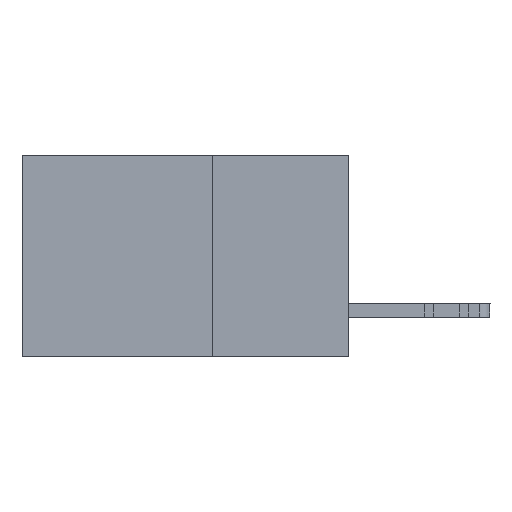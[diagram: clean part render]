
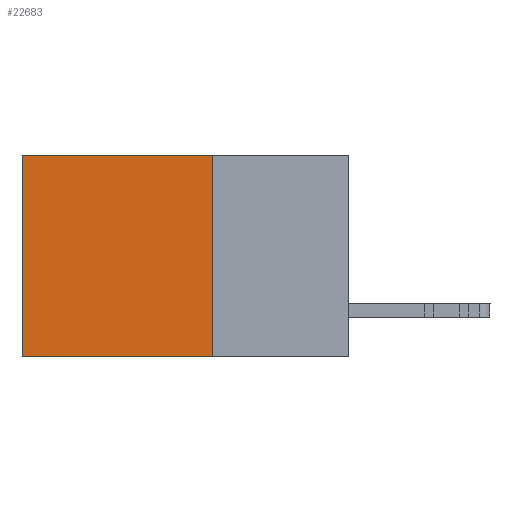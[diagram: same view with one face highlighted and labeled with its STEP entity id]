
A CAD part, left-side view. The second image highlights one B-rep face of the part: STEP entity #22683.
In plain terms, the highlighted planar face has unit normal (-1, 0, 0).
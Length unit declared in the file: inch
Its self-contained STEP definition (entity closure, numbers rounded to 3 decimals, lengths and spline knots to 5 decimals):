
#651 = DIRECTION ( 'NONE',  ( 0., 0., -1. ) ) ;
#718 = ORIENTED_EDGE ( 'NONE', *, *, #1273, .F. ) ;
#754 = VERTEX_POINT ( 'NONE', #18530 ) ;
#1040 = EDGE_CURVE ( 'NONE', #19970, #754, #9761, .T. ) ;
#1273 = EDGE_CURVE ( 'NONE', #754, #12053, #20015, .T. ) ;
#4114 = DIRECTION ( 'NONE',  ( 0., 1., 0. ) ) ;
#4291 = EDGE_LOOP ( 'NONE', ( #14444, #718, #12675, #13994 ) ) ;
#4366 = VECTOR ( 'NONE', #651, 39.37008 ) ;
#4708 = CARTESIAN_POINT ( 'NONE',  ( 0.2615, 0.6, 0. ) ) ;
#5606 = VERTEX_POINT ( 'NONE', #4708 ) ;
#6152 = CARTESIAN_POINT ( 'NONE',  ( 0.2615, 0.25, 0. ) ) ;
#7770 = CARTESIAN_POINT ( 'NONE',  ( 0.2615, 0.6, -0.37 ) ) ;
#8842 = EDGE_CURVE ( 'NONE', #5606, #12053, #23587, .T. ) ;
#9646 = EDGE_CURVE ( 'NONE', #19970, #5606, #21411, .T. ) ;
#9761 = LINE ( 'NONE', #25579, #4366 ) ;
#11056 = DIRECTION ( 'NONE',  ( 1., 0., 0. ) ) ;
#12053 = VERTEX_POINT ( 'NONE', #12537 ) ;
#12537 = CARTESIAN_POINT ( 'NONE',  ( 0.2615, 0.6, -0.37 ) ) ;
#12675 = ORIENTED_EDGE ( 'NONE', *, *, #1040, .F. ) ;
#13994 = ORIENTED_EDGE ( 'NONE', *, *, #9646, .T. ) ;
#14444 = ORIENTED_EDGE ( 'NONE', *, *, #8842, .T. ) ;
#14761 = VECTOR ( 'NONE', #19739, 39.37008 ) ;
#17314 = AXIS2_PLACEMENT_3D ( 'NONE', #22886, #11056, #24857 ) ;
#17716 = FACE_OUTER_BOUND ( 'NONE', #4291, .T. ) ;
#18530 = CARTESIAN_POINT ( 'NONE',  ( 0.2615, 0.25, -0.37 ) ) ;
#18763 = CARTESIAN_POINT ( 'NONE',  ( 0.2615, 0.25, -0.37 ) ) ;
#18962 = PLANE ( 'NONE',  #17314 ) ;
#19609 = VECTOR ( 'NONE', #21716, 39.37008 ) ;
#19739 = DIRECTION ( 'NONE',  ( 0., 1., 0. ) ) ;
#19970 = VERTEX_POINT ( 'NONE', #25408 ) ;
#20015 = LINE ( 'NONE', #18763, #14761 ) ;
#20174 = VECTOR ( 'NONE', #4114, 39.37008 ) ;
#21411 = LINE ( 'NONE', #6152, #20174 ) ;
#21716 = DIRECTION ( 'NONE',  ( 0., 0., -1. ) ) ;
#22683 = ADVANCED_FACE ( 'NONE', ( #17716 ), #18962, .F. ) ;
#22886 = CARTESIAN_POINT ( 'NONE',  ( 0.2615, 0.25, -0.37 ) ) ;
#23587 = LINE ( 'NONE', #7770, #19609 ) ;
#24857 = DIRECTION ( 'NONE',  ( 0., 0., -1. ) ) ;
#25408 = CARTESIAN_POINT ( 'NONE',  ( 0.2615, 0.25, 0. ) ) ;
#25579 = CARTESIAN_POINT ( 'NONE',  ( 0.2615, 0.25, -0.37 ) ) ;
